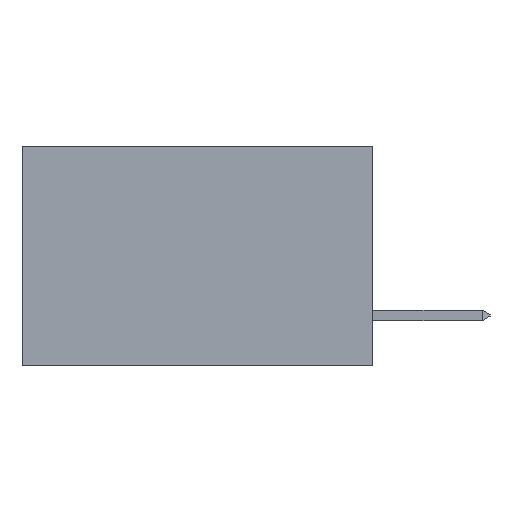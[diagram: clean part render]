
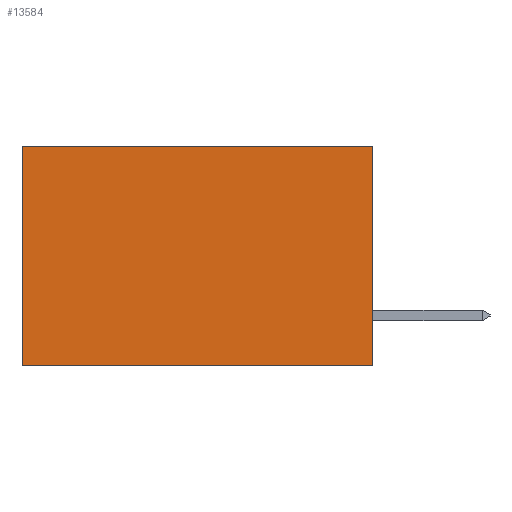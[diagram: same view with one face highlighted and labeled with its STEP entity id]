
A CAD part, left-side view. The second image highlights one B-rep face of the part: STEP entity #13584.
In plain terms, the highlighted planar face has unit normal (-1, 0, 0).
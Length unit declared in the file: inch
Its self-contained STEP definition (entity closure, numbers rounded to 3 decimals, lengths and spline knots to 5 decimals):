
#21 = ORIENTED_EDGE ( 'NONE', *, *, #3165, .F. ) ;
#325 = ORIENTED_EDGE ( 'NONE', *, *, #1109, .T. ) ;
#867 = CARTESIAN_POINT ( 'NONE',  ( 0.277, 0.59, 0. ) ) ;
#1109 = EDGE_CURVE ( 'NONE', #7364, #6420, #11694, .T. ) ;
#1261 = DIRECTION ( 'NONE',  ( 0., 0., -1. ) ) ;
#2012 = AXIS2_PLACEMENT_3D ( 'NONE', #11362, #5793, #13597 ) ;
#2164 = CARTESIAN_POINT ( 'NONE',  ( 0.277, 0., 0. ) ) ;
#2266 = ORIENTED_EDGE ( 'NONE', *, *, #10184, .T. ) ;
#2998 = VECTOR ( 'NONE', #12433, 39.37008 ) ;
#3165 = EDGE_CURVE ( 'NONE', #7364, #3772, #7140, .T. ) ;
#3320 = CARTESIAN_POINT ( 'NONE',  ( 0.277, 0., -0.37 ) ) ;
#3772 = VERTEX_POINT ( 'NONE', #11854 ) ;
#4082 = VECTOR ( 'NONE', #9121, 39.37008 ) ;
#4616 = PLANE ( 'NONE',  #2012 ) ;
#5132 = EDGE_LOOP ( 'NONE', ( #2266, #8376, #21, #325 ) ) ;
#5727 = FACE_OUTER_BOUND ( 'NONE', #5132, .T. ) ;
#5793 = DIRECTION ( 'NONE',  ( 1., 0., 0. ) ) ;
#6420 = VERTEX_POINT ( 'NONE', #867 ) ;
#7140 = LINE ( 'NONE', #12892, #4082 ) ;
#7364 = VERTEX_POINT ( 'NONE', #2164 ) ;
#7799 = DIRECTION ( 'NONE',  ( 0., 1., 0. ) ) ;
#8293 = EDGE_CURVE ( 'NONE', #3772, #11610, #14425, .T. ) ;
#8376 = ORIENTED_EDGE ( 'NONE', *, *, #8293, .F. ) ;
#8490 = CARTESIAN_POINT ( 'NONE',  ( 0.277, 0.59, -0.37 ) ) ;
#9121 = DIRECTION ( 'NONE',  ( 0., 0., -1. ) ) ;
#9791 = CARTESIAN_POINT ( 'NONE',  ( 0.277, 0., 0. ) ) ;
#9898 = LINE ( 'NONE', #11515, #12503 ) ;
#10184 = EDGE_CURVE ( 'NONE', #6420, #11610, #9898, .T. ) ;
#11362 = CARTESIAN_POINT ( 'NONE',  ( 0.277, 0., -0.37 ) ) ;
#11486 = VECTOR ( 'NONE', #7799, 39.37008 ) ;
#11515 = CARTESIAN_POINT ( 'NONE',  ( 0.277, 0.59, -0.37 ) ) ;
#11610 = VERTEX_POINT ( 'NONE', #8490 ) ;
#11694 = LINE ( 'NONE', #9791, #2998 ) ;
#11854 = CARTESIAN_POINT ( 'NONE',  ( 0.277, 0., -0.37 ) ) ;
#12433 = DIRECTION ( 'NONE',  ( 0., 1., 0. ) ) ;
#12503 = VECTOR ( 'NONE', #1261, 39.37008 ) ;
#12892 = CARTESIAN_POINT ( 'NONE',  ( 0.277, 0., -0.37 ) ) ;
#13584 = ADVANCED_FACE ( 'NONE', ( #5727 ), #4616, .F. ) ;
#13597 = DIRECTION ( 'NONE',  ( 0., 0., -1. ) ) ;
#14425 = LINE ( 'NONE', #3320, #11486 ) ;
